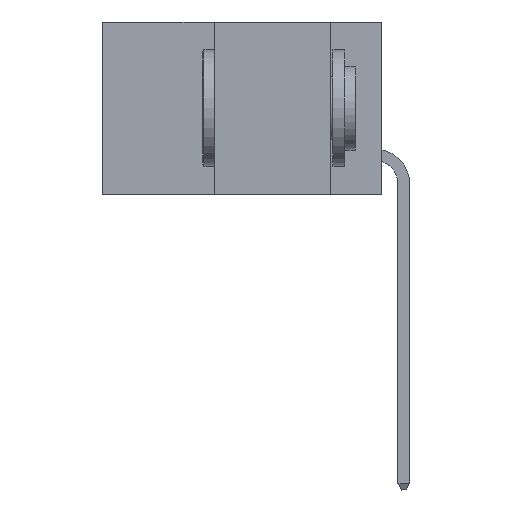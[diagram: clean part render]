
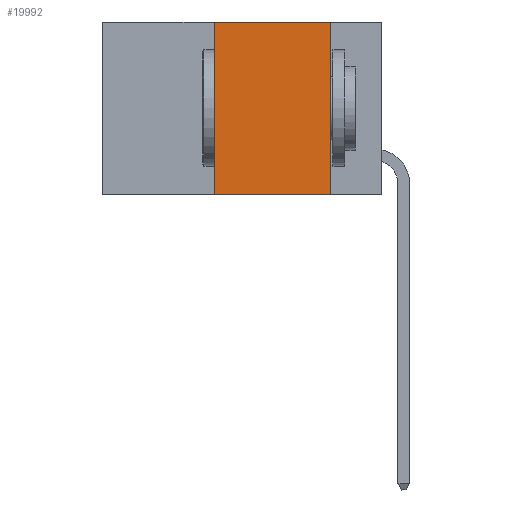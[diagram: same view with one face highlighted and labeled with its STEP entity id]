
A CAD part, left-side view. The second image highlights one B-rep face of the part: STEP entity #19992.
In plain terms, the highlighted planar face has unit normal (-1, 0, 0).
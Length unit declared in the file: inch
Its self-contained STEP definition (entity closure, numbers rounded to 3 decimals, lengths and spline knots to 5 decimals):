
#2047 = VERTEX_POINT ( 'NONE', #8138 ) ;
#5118 = LINE ( 'NONE', #16582, #25332 ) ;
#8138 = CARTESIAN_POINT ( 'NONE',  ( 0., 0.36, 0. ) ) ;
#8885 = EDGE_CURVE ( 'NONE', #12636, #20562, #41740, .T. ) ;
#10776 = DIRECTION ( 'NONE',  ( 0., 0., 1. ) ) ;
#11593 = LINE ( 'NONE', #42611, #40593 ) ;
#12636 = VERTEX_POINT ( 'NONE', #27717 ) ;
#13368 = LINE ( 'NONE', #33460, #33466 ) ;
#13443 = VERTEX_POINT ( 'NONE', #32097 ) ;
#15681 = CARTESIAN_POINT ( 'NONE',  ( 0., 0.6, 0. ) ) ;
#16137 = ORIENTED_EDGE ( 'NONE', *, *, #35007, .F. ) ;
#16582 = CARTESIAN_POINT ( 'NONE',  ( 0., 0.11, 0. ) ) ;
#19497 = DIRECTION ( 'NONE',  ( 0., 0., -1. ) ) ;
#19992 = ADVANCED_FACE ( 'NONE', ( #45135 ), #38343, .F. ) ;
#20562 = VERTEX_POINT ( 'NONE', #48816 ) ;
#21582 = VECTOR ( 'NONE', #42409, 39.37008 ) ;
#21614 = ORIENTED_EDGE ( 'NONE', *, *, #8885, .T. ) ;
#25332 = VECTOR ( 'NONE', #43044, 39.37008 ) ;
#27717 = CARTESIAN_POINT ( 'NONE',  ( 0., 0.36, -0.37 ) ) ;
#29575 = AXIS2_PLACEMENT_3D ( 'NONE', #15681, #30704, #19497 ) ;
#30176 = EDGE_CURVE ( 'NONE', #12636, #2047, #13368, .T. ) ;
#30704 = DIRECTION ( 'NONE',  ( 1., 0., 0. ) ) ;
#31033 = EDGE_LOOP ( 'NONE', ( #16137, #34714, #48131, #21614 ) ) ;
#32097 = CARTESIAN_POINT ( 'NONE',  ( 0., 0.11, 0. ) ) ;
#33460 = CARTESIAN_POINT ( 'NONE',  ( 0., 0.36, 0. ) ) ;
#33466 = VECTOR ( 'NONE', #10776, 39.37008 ) ;
#34714 = ORIENTED_EDGE ( 'NONE', *, *, #44748, .F. ) ;
#35007 = EDGE_CURVE ( 'NONE', #13443, #20562, #5118, .T. ) ;
#38343 = PLANE ( 'NONE',  #29575 ) ;
#38583 = CARTESIAN_POINT ( 'NONE',  ( 0., 0.6, -0.37 ) ) ;
#40593 = VECTOR ( 'NONE', #46432, 39.37008 ) ;
#41740 = LINE ( 'NONE', #38583, #21582 ) ;
#42409 = DIRECTION ( 'NONE',  ( 0., -1., 0. ) ) ;
#42611 = CARTESIAN_POINT ( 'NONE',  ( 0., 0.6, 0. ) ) ;
#43044 = DIRECTION ( 'NONE',  ( 0., 0., -1. ) ) ;
#44748 = EDGE_CURVE ( 'NONE', #2047, #13443, #11593, .T. ) ;
#45135 = FACE_OUTER_BOUND ( 'NONE', #31033, .T. ) ;
#46432 = DIRECTION ( 'NONE',  ( 0., -1., 0. ) ) ;
#48131 = ORIENTED_EDGE ( 'NONE', *, *, #30176, .F. ) ;
#48816 = CARTESIAN_POINT ( 'NONE',  ( 0., 0.11, -0.37 ) ) ;
